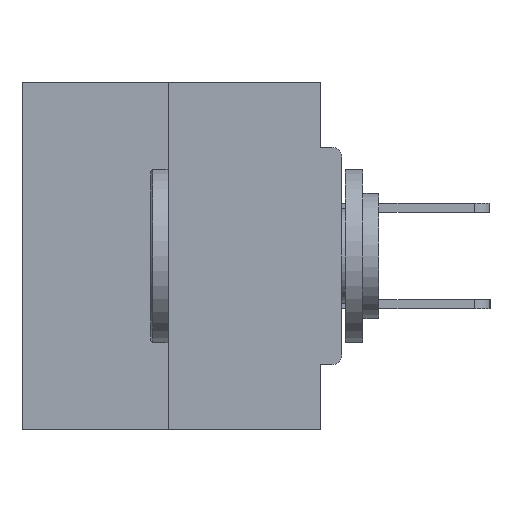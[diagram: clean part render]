
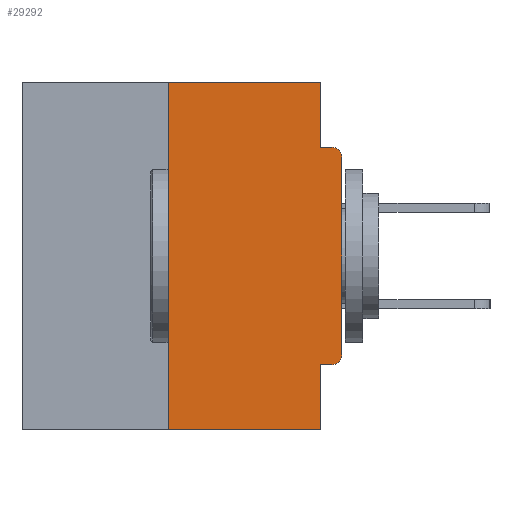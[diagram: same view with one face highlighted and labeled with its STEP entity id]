
A CAD part, left-side view. The second image highlights one B-rep face of the part: STEP entity #29292.
In plain terms, the highlighted planar face has unit normal (-1, 0, 0).
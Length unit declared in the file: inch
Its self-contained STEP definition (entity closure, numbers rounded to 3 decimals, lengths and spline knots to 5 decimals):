
#461 = VERTEX_POINT ( 'NONE', #5108 ) ;
#537 = DIRECTION ( 'NONE',  ( 0., 0., -1. ) ) ;
#826 = ORIENTED_EDGE ( 'NONE', *, *, #25102, .F. ) ;
#1248 = CIRCLE ( 'NONE', #7686, 0.015 ) ;
#1895 = VERTEX_POINT ( 'NONE', #15502 ) ;
#2475 = ORIENTED_EDGE ( 'NONE', *, *, #11954, .T. ) ;
#2805 = DIRECTION ( 'NONE',  ( 0., -1., 0. ) ) ;
#2820 = CARTESIAN_POINT ( 'NONE',  ( 0., 0.25, -0.5 ) ) ;
#2895 = EDGE_CURVE ( 'NONE', #1895, #24481, #5705, .T. ) ;
#4055 = CARTESIAN_POINT ( 'NONE',  ( 0., 0.015, -0.1085 ) ) ;
#4163 = VECTOR ( 'NONE', #18033, 39.37008 ) ;
#4386 = CARTESIAN_POINT ( 'NONE',  ( 0., 0.031, 0. ) ) ;
#4970 = DIRECTION ( 'NONE',  ( 0., 1., 0. ) ) ;
#5108 = CARTESIAN_POINT ( 'NONE',  ( 0., 0.031, -0.0935 ) ) ;
#5705 = LINE ( 'NONE', #12750, #25198 ) ;
#6705 = ORIENTED_EDGE ( 'NONE', *, *, #16820, .F. ) ;
#6796 = ORIENTED_EDGE ( 'NONE', *, *, #8265, .F. ) ;
#6857 = DIRECTION ( 'NONE',  ( 0., 0., -1. ) ) ;
#6882 = CARTESIAN_POINT ( 'NONE',  ( 0., 0.25, 0. ) ) ;
#6937 = FACE_OUTER_BOUND ( 'NONE', #12956, .T. ) ;
#7208 = DIRECTION ( 'NONE',  ( 0., 0., -1. ) ) ;
#7303 = CARTESIAN_POINT ( 'NONE',  ( 0., 0.46, -0.5 ) ) ;
#7549 = DIRECTION ( 'NONE',  ( 0., 0., 1. ) ) ;
#7590 = LINE ( 'NONE', #7932, #35273 ) ;
#7636 = VERTEX_POINT ( 'NONE', #33363 ) ;
#7686 = AXIS2_PLACEMENT_3D ( 'NONE', #13519, #22009, #27661 ) ;
#7760 = DIRECTION ( 'NONE',  ( 1., 0., 0. ) ) ;
#7932 = CARTESIAN_POINT ( 'NONE',  ( 0., 0., -0.0935 ) ) ;
#8184 = EDGE_CURVE ( 'NONE', #11255, #18232, #33571, .T. ) ;
#8265 = EDGE_CURVE ( 'NONE', #7636, #15093, #12763, .T. ) ;
#8321 = CARTESIAN_POINT ( 'NONE',  ( 0., 0.031, -0.5 ) ) ;
#8621 = CIRCLE ( 'NONE', #16916, 0.015 ) ;
#8882 = CARTESIAN_POINT ( 'NONE',  ( 0., 0.031, 0. ) ) ;
#10537 = CARTESIAN_POINT ( 'NONE',  ( 0., 0.46, 0. ) ) ;
#10610 = CARTESIAN_POINT ( 'NONE',  ( 0., 0.015, -0.4065 ) ) ;
#10789 = VECTOR ( 'NONE', #537, 39.37008 ) ;
#11184 = CARTESIAN_POINT ( 'NONE',  ( 0., 0.46, 0. ) ) ;
#11255 = VERTEX_POINT ( 'NONE', #10610 ) ;
#11954 = EDGE_CURVE ( 'NONE', #24481, #15465, #8621, .T. ) ;
#12150 = VECTOR ( 'NONE', #7208, 39.37008 ) ;
#12750 = CARTESIAN_POINT ( 'NONE',  ( 0., 0., 0. ) ) ;
#12763 = LINE ( 'NONE', #11184, #14512 ) ;
#12860 = CARTESIAN_POINT ( 'NONE',  ( 0., 0., -0.1085 ) ) ;
#12956 = EDGE_LOOP ( 'NONE', ( #6796, #826, #32853, #14278, #16063, #21420, #17853, #2475, #6705, #17125 ) ) ;
#12967 = DIRECTION ( 'NONE',  ( 0., 0., -1. ) ) ;
#13519 = CARTESIAN_POINT ( 'NONE',  ( 0., 0.015, -0.3915 ) ) ;
#13598 = CARTESIAN_POINT ( 'NONE',  ( 0., 0., -0.4065 ) ) ;
#14278 = ORIENTED_EDGE ( 'NONE', *, *, #14433, .F. ) ;
#14284 = EDGE_CURVE ( 'NONE', #11255, #1895, #1248, .T. ) ;
#14433 = EDGE_CURVE ( 'NONE', #18232, #22376, #30732, .T. ) ;
#14512 = VECTOR ( 'NONE', #2805, 39.37008 ) ;
#15093 = VERTEX_POINT ( 'NONE', #8882 ) ;
#15465 = VERTEX_POINT ( 'NONE', #24214 ) ;
#15502 = CARTESIAN_POINT ( 'NONE',  ( 0., 0., -0.3915 ) ) ;
#15988 = CARTESIAN_POINT ( 'NONE',  ( 0., 0.031, -0.4065 ) ) ;
#16063 = ORIENTED_EDGE ( 'NONE', *, *, #8184, .F. ) ;
#16224 = PLANE ( 'NONE',  #32894 ) ;
#16820 = EDGE_CURVE ( 'NONE', #461, #15465, #7590, .T. ) ;
#16916 = AXIS2_PLACEMENT_3D ( 'NONE', #4055, #26208, #6857 ) ;
#17125 = ORIENTED_EDGE ( 'NONE', *, *, #28540, .F. ) ;
#17705 = VERTEX_POINT ( 'NONE', #2820 ) ;
#17853 = ORIENTED_EDGE ( 'NONE', *, *, #2895, .T. ) ;
#18033 = DIRECTION ( 'NONE',  ( 0., 0., 1. ) ) ;
#18232 = VERTEX_POINT ( 'NONE', #15988 ) ;
#18834 = DIRECTION ( 'NONE',  ( 0., -1., 0. ) ) ;
#19534 = LINE ( 'NONE', #4386, #12150 ) ;
#20301 = VECTOR ( 'NONE', #29188, 39.37008 ) ;
#21420 = ORIENTED_EDGE ( 'NONE', *, *, #14284, .T. ) ;
#22009 = DIRECTION ( 'NONE',  ( -1., 0., 0. ) ) ;
#22376 = VERTEX_POINT ( 'NONE', #23949 ) ;
#23949 = CARTESIAN_POINT ( 'NONE',  ( 0., 0.031, -0.5 ) ) ;
#24214 = CARTESIAN_POINT ( 'NONE',  ( 0., 0.015, -0.0935 ) ) ;
#24481 = VERTEX_POINT ( 'NONE', #12860 ) ;
#25102 = EDGE_CURVE ( 'NONE', #17705, #7636, #33645, .T. ) ;
#25198 = VECTOR ( 'NONE', #7549, 39.37008 ) ;
#26208 = DIRECTION ( 'NONE',  ( -1., 0., 0. ) ) ;
#27645 = LINE ( 'NONE', #7303, #20301 ) ;
#27661 = DIRECTION ( 'NONE',  ( 0., 0., -1. ) ) ;
#27919 = VECTOR ( 'NONE', #4970, 39.37008 ) ;
#28540 = EDGE_CURVE ( 'NONE', #15093, #461, #19534, .T. ) ;
#29188 = DIRECTION ( 'NONE',  ( 0., -1., 0. ) ) ;
#29292 = ADVANCED_FACE ( 'NONE', ( #6937 ), #16224, .F. ) ;
#30732 = LINE ( 'NONE', #8321, #10789 ) ;
#32853 = ORIENTED_EDGE ( 'NONE', *, *, #34080, .T. ) ;
#32894 = AXIS2_PLACEMENT_3D ( 'NONE', #10537, #7760, #12967 ) ;
#33363 = CARTESIAN_POINT ( 'NONE',  ( 0., 0.25, 0. ) ) ;
#33571 = LINE ( 'NONE', #13598, #27919 ) ;
#33645 = LINE ( 'NONE', #6882, #4163 ) ;
#34080 = EDGE_CURVE ( 'NONE', #17705, #22376, #27645, .T. ) ;
#35273 = VECTOR ( 'NONE', #18834, 39.37008 ) ;
